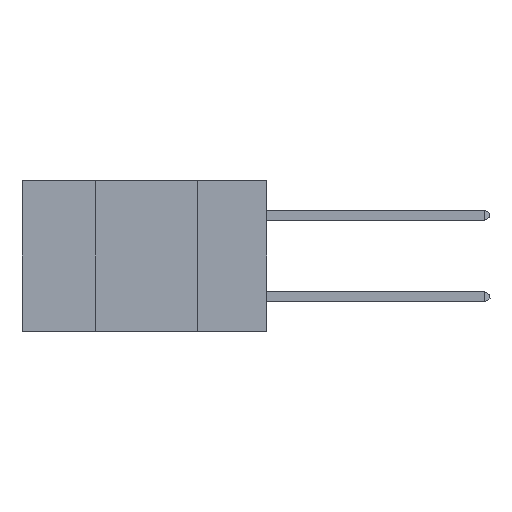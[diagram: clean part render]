
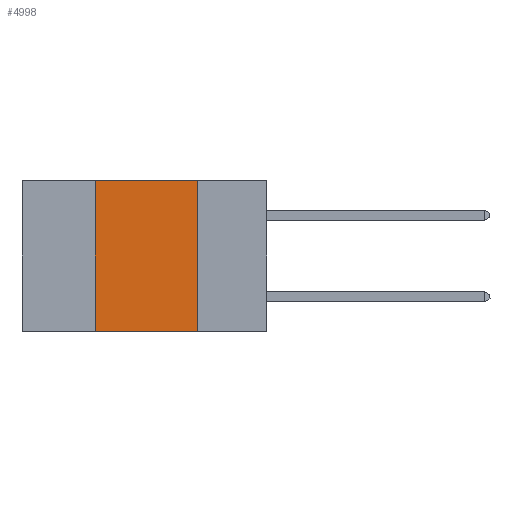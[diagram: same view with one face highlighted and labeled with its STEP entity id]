
A CAD part, left-side view. The second image highlights one B-rep face of the part: STEP entity #4998.
In plain terms, the highlighted planar face has unit normal (-1, 0, 0).
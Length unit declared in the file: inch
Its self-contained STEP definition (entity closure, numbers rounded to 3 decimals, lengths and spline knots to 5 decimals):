
#1290 = ORIENTED_EDGE ( 'NONE', *, *, #5099, .T. ) ;
#1434 = EDGE_CURVE ( 'NONE', #11941, #9780, #5327, .T. ) ;
#1755 = DIRECTION ( 'NONE',  ( 0., -1., 0. ) ) ;
#1947 = DIRECTION ( 'NONE',  ( 0., 0., 1. ) ) ;
#2814 = DIRECTION ( 'NONE',  ( 0., -1., 0. ) ) ;
#3033 = EDGE_CURVE ( 'NONE', #5101, #11941, #6974, .T. ) ;
#3802 = DIRECTION ( 'NONE',  ( 1., 0., 0. ) ) ;
#4793 = CARTESIAN_POINT ( 'NONE',  ( 0., 0.42, -0.37 ) ) ;
#4998 = ADVANCED_FACE ( 'NONE', ( #10135 ), #9651, .F. ) ;
#5099 = EDGE_CURVE ( 'NONE', #10482, #9780, #10845, .T. ) ;
#5101 = VERTEX_POINT ( 'NONE', #14324 ) ;
#5327 = LINE ( 'NONE', #5983, #13789 ) ;
#5983 = CARTESIAN_POINT ( 'NONE',  ( 0., 0.17, 0. ) ) ;
#6974 = LINE ( 'NONE', #8542, #12343 ) ;
#7015 = ORIENTED_EDGE ( 'NONE', *, *, #11679, .F. ) ;
#7483 = EDGE_LOOP ( 'NONE', ( #10456, #9588, #7015, #1290 ) ) ;
#8412 = CARTESIAN_POINT ( 'NONE',  ( 0., 0.6, 0. ) ) ;
#8542 = CARTESIAN_POINT ( 'NONE',  ( 0., 0.6, 0. ) ) ;
#8735 = CARTESIAN_POINT ( 'NONE',  ( 0., 0.17, -0.37 ) ) ;
#9067 = AXIS2_PLACEMENT_3D ( 'NONE', #8412, #3802, #10657 ) ;
#9588 = ORIENTED_EDGE ( 'NONE', *, *, #3033, .F. ) ;
#9651 = PLANE ( 'NONE',  #9067 ) ;
#9780 = VERTEX_POINT ( 'NONE', #8735 ) ;
#9959 = CARTESIAN_POINT ( 'NONE',  ( 0., 0.17, 0. ) ) ;
#10135 = FACE_OUTER_BOUND ( 'NONE', #7483, .T. ) ;
#10456 = ORIENTED_EDGE ( 'NONE', *, *, #1434, .F. ) ;
#10482 = VERTEX_POINT ( 'NONE', #4793 ) ;
#10586 = DIRECTION ( 'NONE',  ( 0., 0., -1. ) ) ;
#10657 = DIRECTION ( 'NONE',  ( 0., 0., -1. ) ) ;
#10845 = LINE ( 'NONE', #10999, #12828 ) ;
#10999 = CARTESIAN_POINT ( 'NONE',  ( 0., 0.6, -0.37 ) ) ;
#11263 = LINE ( 'NONE', #13309, #13253 ) ;
#11679 = EDGE_CURVE ( 'NONE', #10482, #5101, #11263, .T. ) ;
#11941 = VERTEX_POINT ( 'NONE', #9959 ) ;
#12343 = VECTOR ( 'NONE', #1755, 39.37008 ) ;
#12828 = VECTOR ( 'NONE', #2814, 39.37008 ) ;
#13253 = VECTOR ( 'NONE', #1947, 39.37008 ) ;
#13309 = CARTESIAN_POINT ( 'NONE',  ( 0., 0.42, 0. ) ) ;
#13789 = VECTOR ( 'NONE', #10586, 39.37008 ) ;
#14324 = CARTESIAN_POINT ( 'NONE',  ( 0., 0.42, 0. ) ) ;
